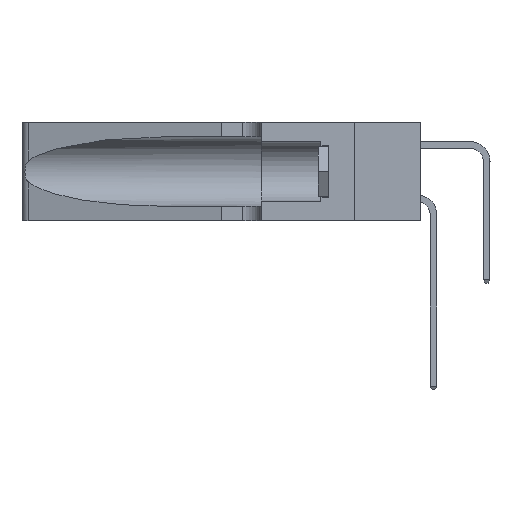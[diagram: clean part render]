
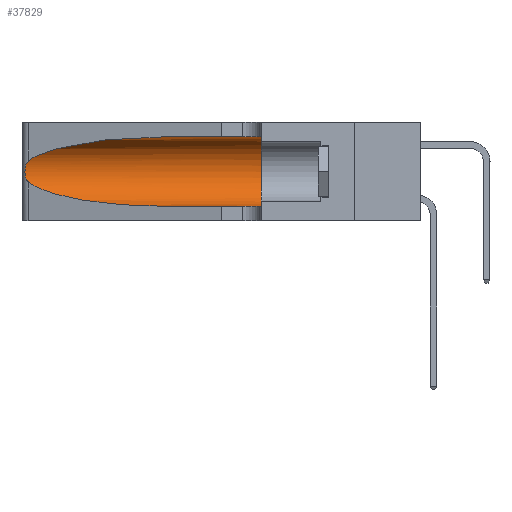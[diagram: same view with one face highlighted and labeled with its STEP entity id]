
A CAD part, left-side view. The second image highlights one B-rep face of the part: STEP entity #37829.
In plain terms, the highlighted cylindrical face has radius 3.308 mm (diameter 6.617 mm), a partial arc.
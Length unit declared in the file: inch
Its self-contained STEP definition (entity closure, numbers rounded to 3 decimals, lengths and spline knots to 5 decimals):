
#574 = DIRECTION ( 'NONE',  ( 0., -1., 0. ) ) ;
#1383 =( BOUNDED_CURVE ( )  B_SPLINE_CURVE ( 3, ( #32722, #38662, #26660, #35767 ),
 .UNSPECIFIED., .F., .F. ) 
 B_SPLINE_CURVE_WITH_KNOTS ( ( 4, 4 ),
 ( 1.5708, 2.84003 ),
 .UNSPECIFIED. ) 
 CURVE ( )  GEOMETRIC_REPRESENTATION_ITEM ( )  RATIONAL_B_SPLINE_CURVE ( ( 1., 0.87, 0.87, 1. ) ) 
 REPRESENTATION_ITEM ( '' )  );
#2165 = CIRCLE ( 'NONE', #10326, 0.13025 ) ;
#2433 = CARTESIAN_POINT ( 'NONE',  ( 0.25487, 1.22718, 0.14631 ) ) ;
#2577 =( BOUNDED_CURVE ( )  B_SPLINE_CURVE ( 3, ( #2433, #23823, #5480, #26894 ),
 .UNSPECIFIED., .F., .F. ) 
 B_SPLINE_CURVE_WITH_KNOTS ( ( 4, 4 ),
 ( 3.44316, 4.71239 ),
 .UNSPECIFIED. ) 
 CURVE ( )  GEOMETRIC_REPRESENTATION_ITEM ( )  RATIONAL_B_SPLINE_CURVE ( ( 1., 0.87, 0.87, 1. ) ) 
 REPRESENTATION_ITEM ( '' )  );
#2901 = CARTESIAN_POINT ( 'NONE',  ( 0.26075, 1.23896, 0.178 ) ) ;
#4091 = AXIS2_PLACEMENT_3D ( 'NONE', #9743, #574, #25021 ) ;
#4206 = ORIENTED_EDGE ( 'NONE', *, *, #9894, .F. ) ;
#4687 = EDGE_CURVE ( 'NONE', #19646, #36081, #1383, .T. ) ;
#5480 = CARTESIAN_POINT ( 'NONE',  ( 0.18966, 0.96281, 0.05475 ) ) ;
#5511 = LINE ( 'NONE', #33039, #21802 ) ;
#5979 = CARTESIAN_POINT ( 'NONE',  ( 0.25856, 1.23593, 0.16098 ) ) ;
#7865 = DIRECTION ( 'NONE',  ( 0., -1., 0. ) ) ;
#9048 = CARTESIAN_POINT ( 'NONE',  ( 0.25639, 1.23186, 0.15144 ) ) ;
#9691 = VERTEX_POINT ( 'NONE', #34932 ) ;
#9743 = CARTESIAN_POINT ( 'NONE',  ( 0.1305, 1.61858, 0.185 ) ) ;
#9894 = EDGE_CURVE ( 'NONE', #19646, #15929, #5511, .T. ) ;
#9953 = EDGE_CURVE ( 'NONE', #36081, #25220, #17749, .T. ) ;
#10326 = AXIS2_PLACEMENT_3D ( 'NONE', #13434, #34744, #16563 ) ;
#10858 = VECTOR ( 'NONE', #7865, 39.37008 ) ;
#12101 = CARTESIAN_POINT ( 'NONE',  ( 0.25487, 1.22718, 0.14631 ) ) ;
#12567 = ORIENTED_EDGE ( 'NONE', *, *, #4687, .T. ) ;
#13434 = CARTESIAN_POINT ( 'NONE',  ( 0.1305, 0.35, 0.185 ) ) ;
#14796 = DIRECTION ( 'NONE',  ( 0., -1., 0. ) ) ;
#15071 = CARTESIAN_POINT ( 'NONE',  ( 0.25639, 1.23184, 0.21858 ) ) ;
#15725 = ORIENTED_EDGE ( 'NONE', *, *, #16179, .F. ) ;
#15929 = VERTEX_POINT ( 'NONE', #36604 ) ;
#16179 = EDGE_CURVE ( 'NONE', #15929, #9691, #2165, .T. ) ;
#16563 = DIRECTION ( 'NONE',  ( 0., 0., 1. ) ) ;
#17749 = B_SPLINE_CURVE_WITH_KNOTS ( 'NONE', 3,
 ( #30273, #33296, #15071, #36334, #18164, #39354, #21237, #2901, #24311, #5979, #27366, #9048, #30410, #12101 ),
 .UNSPECIFIED., .F., .F.,
 ( 4, 2, 2, 2, 2, 2, 4 ),
 ( 0., 0.00027, 0.00053, 0.00107, 0.0016, 0.00187, 0.00214 ),
 .UNSPECIFIED. ) ;
#17763 = EDGE_CURVE ( 'NONE', #25220, #26718, #2577, .T. ) ;
#18137 = ORIENTED_EDGE ( 'NONE', *, *, #39241, .T. ) ;
#18164 = CARTESIAN_POINT ( 'NONE',  ( 0.25854, 1.2359, 0.20912 ) ) ;
#19025 = LINE ( 'NONE', #23113, #10858 ) ;
#19212 = ORIENTED_EDGE ( 'NONE', *, *, #9953, .T. ) ;
#19646 = VERTEX_POINT ( 'NONE', #20387 ) ;
#20387 = CARTESIAN_POINT ( 'NONE',  ( 0.1305, 0.72297, 0.31525 ) ) ;
#21237 = CARTESIAN_POINT ( 'NONE',  ( 0.26075, 1.23896, 0.19203 ) ) ;
#21802 = VECTOR ( 'NONE', #14796, 39.37008 ) ;
#22010 = FACE_OUTER_BOUND ( 'NONE', #32463, .T. ) ;
#23113 = CARTESIAN_POINT ( 'NONE',  ( 0.1305, 1.61858, 0.05475 ) ) ;
#23823 = CARTESIAN_POINT ( 'NONE',  ( 0.2373, 1.15595, 0.08982 ) ) ;
#24311 = CARTESIAN_POINT ( 'NONE',  ( 0.26017, 1.23833, 0.17102 ) ) ;
#25021 = DIRECTION ( 'NONE',  ( 0., 0., -1. ) ) ;
#25220 = VERTEX_POINT ( 'NONE', #25921 ) ;
#25921 = CARTESIAN_POINT ( 'NONE',  ( 0.25487, 1.22718, 0.14631 ) ) ;
#26660 = CARTESIAN_POINT ( 'NONE',  ( 0.2373, 1.15595, 0.28018 ) ) ;
#26718 = VERTEX_POINT ( 'NONE', #28045 ) ;
#26894 = CARTESIAN_POINT ( 'NONE',  ( 0.1305, 0.72297, 0.05475 ) ) ;
#27366 = CARTESIAN_POINT ( 'NONE',  ( 0.25789, 1.23486, 0.15765 ) ) ;
#28045 = CARTESIAN_POINT ( 'NONE',  ( 0.1305, 0.72297, 0.05475 ) ) ;
#30273 = CARTESIAN_POINT ( 'NONE',  ( 0.25487, 1.22718, 0.22369 ) ) ;
#30410 = CARTESIAN_POINT ( 'NONE',  ( 0.25555, 1.22993, 0.14849 ) ) ;
#32463 = EDGE_LOOP ( 'NONE', ( #12567, #19212, #38533, #18137, #15725, #4206 ) ) ;
#32722 = CARTESIAN_POINT ( 'NONE',  ( 0.1305, 0.72297, 0.31525 ) ) ;
#33039 = CARTESIAN_POINT ( 'NONE',  ( 0.1305, 1.61858, 0.31525 ) ) ;
#33296 = CARTESIAN_POINT ( 'NONE',  ( 0.25555, 1.22994, 0.2215 ) ) ;
#34744 = DIRECTION ( 'NONE',  ( 0., 1., 0. ) ) ;
#34932 = CARTESIAN_POINT ( 'NONE',  ( 0.1305, 0.35, 0.05475 ) ) ;
#35767 = CARTESIAN_POINT ( 'NONE',  ( 0.25487, 1.22718, 0.22369 ) ) ;
#36081 = VERTEX_POINT ( 'NONE', #37678 ) ;
#36334 = CARTESIAN_POINT ( 'NONE',  ( 0.25787, 1.23484, 0.2124 ) ) ;
#36604 = CARTESIAN_POINT ( 'NONE',  ( 0.1305, 0.35, 0.31525 ) ) ;
#37167 = CYLINDRICAL_SURFACE ( 'NONE', #4091, 0.13025 ) ;
#37678 = CARTESIAN_POINT ( 'NONE',  ( 0.25487, 1.22718, 0.22369 ) ) ;
#37829 = ADVANCED_FACE ( 'NONE', ( #22010 ), #37167, .F. ) ;
#38533 = ORIENTED_EDGE ( 'NONE', *, *, #17763, .T. ) ;
#38662 = CARTESIAN_POINT ( 'NONE',  ( 0.18966, 0.96281, 0.31525 ) ) ;
#39241 = EDGE_CURVE ( 'NONE', #26718, #9691, #19025, .T. ) ;
#39354 = CARTESIAN_POINT ( 'NONE',  ( 0.26018, 1.23835, 0.19895 ) ) ;
